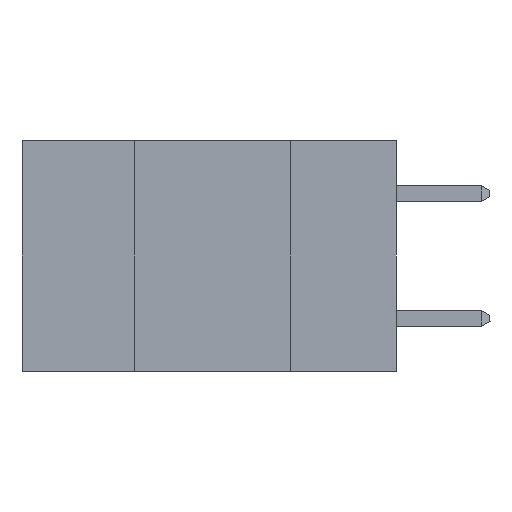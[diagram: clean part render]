
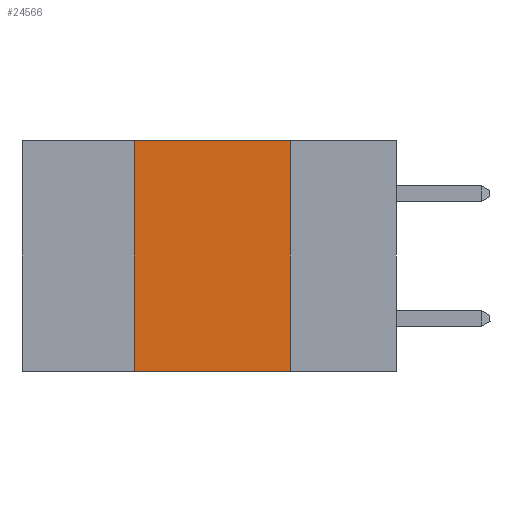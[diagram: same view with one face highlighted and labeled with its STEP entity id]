
A CAD part, left-side view. The second image highlights one B-rep face of the part: STEP entity #24566.
In plain terms, the highlighted planar face has unit normal (-1, 0, 0).
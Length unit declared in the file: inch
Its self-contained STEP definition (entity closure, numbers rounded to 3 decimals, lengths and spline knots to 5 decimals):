
#206 = EDGE_CURVE ( 'NONE', #19794, #5592, #11088, .T. ) ;
#339 = VERTEX_POINT ( 'NONE', #10660 ) ;
#1303 = CARTESIAN_POINT ( 'NONE',  ( 0., 0.6, -0.37 ) ) ;
#2111 = CARTESIAN_POINT ( 'NONE',  ( 0., 0.42, 0. ) ) ;
#2166 = VECTOR ( 'NONE', #16765, 39.37008 ) ;
#5171 = FACE_OUTER_BOUND ( 'NONE', #10151, .T. ) ;
#5592 = VERTEX_POINT ( 'NONE', #2111 ) ;
#6328 = CARTESIAN_POINT ( 'NONE',  ( 0., 0.6, 0. ) ) ;
#8516 = EDGE_CURVE ( 'NONE', #5592, #21101, #26178, .T. ) ;
#10151 = EDGE_LOOP ( 'NONE', ( #15665, #24038, #12684, #17003 ) ) ;
#10240 = CARTESIAN_POINT ( 'NONE',  ( 0., 0.42, 0. ) ) ;
#10308 = LINE ( 'NONE', #25982, #26163 ) ;
#10660 = CARTESIAN_POINT ( 'NONE',  ( 0., 0.17, -0.37 ) ) ;
#10667 = AXIS2_PLACEMENT_3D ( 'NONE', #6328, #13029, #27987 ) ;
#11088 = LINE ( 'NONE', #10240, #21852 ) ;
#12684 = ORIENTED_EDGE ( 'NONE', *, *, #206, .F. ) ;
#12705 = CARTESIAN_POINT ( 'NONE',  ( 0., 0.6, 0. ) ) ;
#13029 = DIRECTION ( 'NONE',  ( 1., 0., 0. ) ) ;
#14707 = LINE ( 'NONE', #1303, #2166 ) ;
#15286 = DIRECTION ( 'NONE',  ( 0., 0., -1. ) ) ;
#15665 = ORIENTED_EDGE ( 'NONE', *, *, #19920, .F. ) ;
#16765 = DIRECTION ( 'NONE',  ( 0., -1., 0. ) ) ;
#16964 = CARTESIAN_POINT ( 'NONE',  ( 0., 0.42, -0.37 ) ) ;
#17003 = ORIENTED_EDGE ( 'NONE', *, *, #17031, .T. ) ;
#17031 = EDGE_CURVE ( 'NONE', #19794, #339, #14707, .T. ) ;
#19794 = VERTEX_POINT ( 'NONE', #16964 ) ;
#19920 = EDGE_CURVE ( 'NONE', #21101, #339, #10308, .T. ) ;
#21101 = VERTEX_POINT ( 'NONE', #21317 ) ;
#21154 = VECTOR ( 'NONE', #27675, 39.37008 ) ;
#21317 = CARTESIAN_POINT ( 'NONE',  ( 0., 0.17, 0. ) ) ;
#21852 = VECTOR ( 'NONE', #26290, 39.37008 ) ;
#24038 = ORIENTED_EDGE ( 'NONE', *, *, #8516, .F. ) ;
#24566 = ADVANCED_FACE ( 'NONE', ( #5171 ), #25899, .F. ) ;
#25899 = PLANE ( 'NONE',  #10667 ) ;
#25982 = CARTESIAN_POINT ( 'NONE',  ( 0., 0.17, 0. ) ) ;
#26163 = VECTOR ( 'NONE', #15286, 39.37008 ) ;
#26178 = LINE ( 'NONE', #12705, #21154 ) ;
#26290 = DIRECTION ( 'NONE',  ( 0., 0., 1. ) ) ;
#27675 = DIRECTION ( 'NONE',  ( 0., -1., 0. ) ) ;
#27987 = DIRECTION ( 'NONE',  ( 0., 0., -1. ) ) ;
